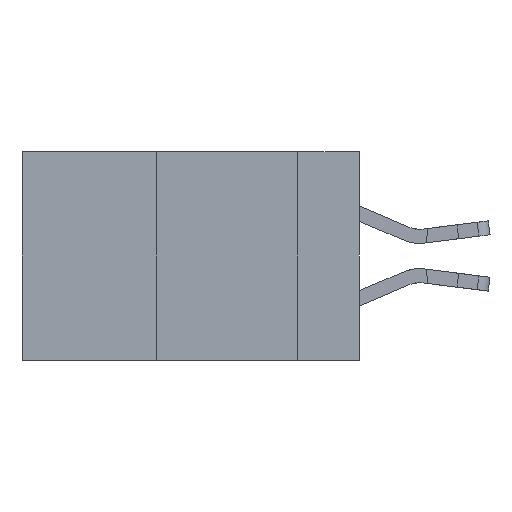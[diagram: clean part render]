
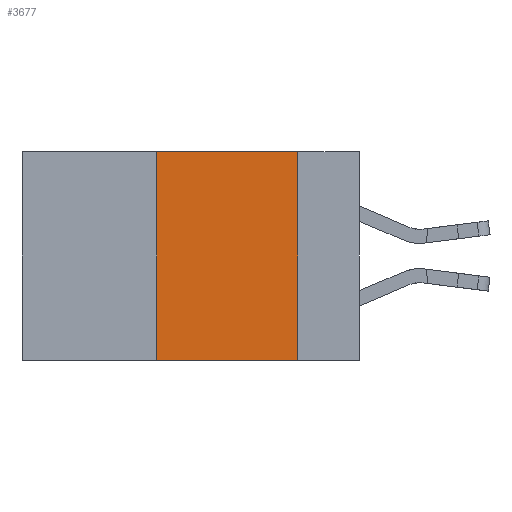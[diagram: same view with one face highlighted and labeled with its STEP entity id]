
A CAD part, left-side view. The second image highlights one B-rep face of the part: STEP entity #3677.
In plain terms, the highlighted planar face has unit normal (-1, 0, 0).
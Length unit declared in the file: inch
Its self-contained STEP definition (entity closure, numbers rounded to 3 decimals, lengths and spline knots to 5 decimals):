
#336 = DIRECTION ( 'NONE',  ( 0., 0., -1. ) ) ;
#443 = VERTEX_POINT ( 'NONE', #14859 ) ;
#959 = VERTEX_POINT ( 'NONE', #4537 ) ;
#1044 = VECTOR ( 'NONE', #10322, 39.37008 ) ;
#1224 = CARTESIAN_POINT ( 'NONE',  ( 0., 0.6, 0. ) ) ;
#1609 = LINE ( 'NONE', #13305, #10139 ) ;
#2152 = ORIENTED_EDGE ( 'NONE', *, *, #14051, .F. ) ;
#2186 = VERTEX_POINT ( 'NONE', #10843 ) ;
#2516 = DIRECTION ( 'NONE',  ( 1., 0., 0. ) ) ;
#2645 = CARTESIAN_POINT ( 'NONE',  ( 0., 0.11, 0. ) ) ;
#3677 = ADVANCED_FACE ( 'NONE', ( #13854 ), #16852, .F. ) ;
#4048 = ORIENTED_EDGE ( 'NONE', *, *, #11908, .F. ) ;
#4267 = LINE ( 'NONE', #2645, #4460 ) ;
#4271 = DIRECTION ( 'NONE',  ( 0., 0., 1. ) ) ;
#4460 = VECTOR ( 'NONE', #336, 39.37008 ) ;
#4537 = CARTESIAN_POINT ( 'NONE',  ( 0., 0.11, 0. ) ) ;
#5078 = LINE ( 'NONE', #6188, #1044 ) ;
#5501 = AXIS2_PLACEMENT_3D ( 'NONE', #1224, #2516, #12824 ) ;
#5552 = CARTESIAN_POINT ( 'NONE',  ( 0., 0.36, 0. ) ) ;
#6188 = CARTESIAN_POINT ( 'NONE',  ( 0., 0.6, 0. ) ) ;
#7283 = EDGE_CURVE ( 'NONE', #959, #2186, #4267, .T. ) ;
#7993 = VECTOR ( 'NONE', #14383, 39.37008 ) ;
#8243 = EDGE_CURVE ( 'NONE', #443, #2186, #14305, .T. ) ;
#8383 = ORIENTED_EDGE ( 'NONE', *, *, #8243, .T. ) ;
#9462 = VERTEX_POINT ( 'NONE', #5552 ) ;
#9485 = EDGE_LOOP ( 'NONE', ( #13302, #2152, #4048, #8383 ) ) ;
#10139 = VECTOR ( 'NONE', #4271, 39.37008 ) ;
#10322 = DIRECTION ( 'NONE',  ( 0., -1., 0. ) ) ;
#10843 = CARTESIAN_POINT ( 'NONE',  ( 0., 0.11, -0.37 ) ) ;
#11652 = CARTESIAN_POINT ( 'NONE',  ( 0., 0.6, -0.37 ) ) ;
#11908 = EDGE_CURVE ( 'NONE', #443, #9462, #1609, .T. ) ;
#12824 = DIRECTION ( 'NONE',  ( 0., 0., -1. ) ) ;
#13302 = ORIENTED_EDGE ( 'NONE', *, *, #7283, .F. ) ;
#13305 = CARTESIAN_POINT ( 'NONE',  ( 0., 0.36, 0. ) ) ;
#13854 = FACE_OUTER_BOUND ( 'NONE', #9485, .T. ) ;
#14051 = EDGE_CURVE ( 'NONE', #9462, #959, #5078, .T. ) ;
#14305 = LINE ( 'NONE', #11652, #7993 ) ;
#14383 = DIRECTION ( 'NONE',  ( 0., -1., 0. ) ) ;
#14859 = CARTESIAN_POINT ( 'NONE',  ( 0., 0.36, -0.37 ) ) ;
#16852 = PLANE ( 'NONE',  #5501 ) ;
